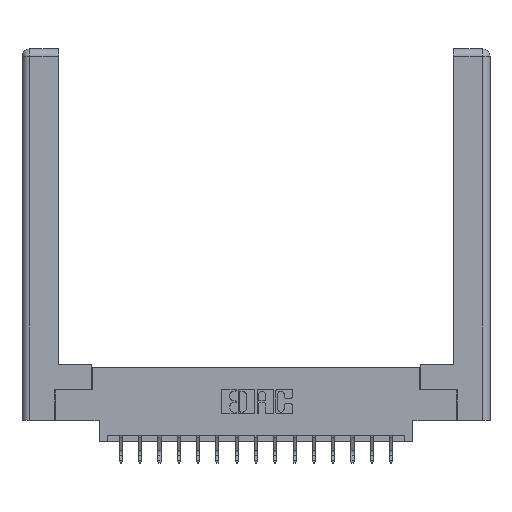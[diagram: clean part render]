
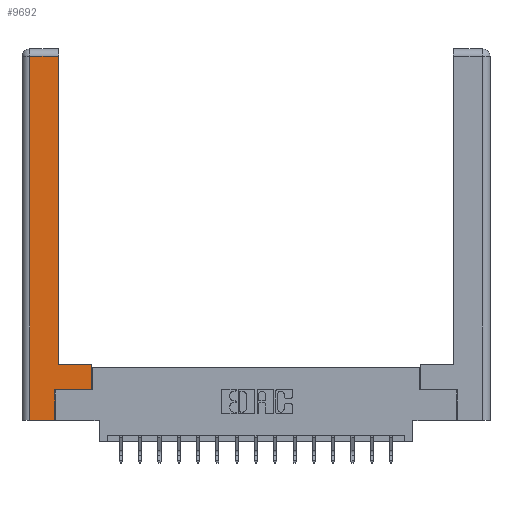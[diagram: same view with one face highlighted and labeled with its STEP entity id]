
A CAD part, top view. The second image highlights one B-rep face of the part: STEP entity #9692.
In plain terms, the highlighted planar face has unit normal (0, 0, 1).
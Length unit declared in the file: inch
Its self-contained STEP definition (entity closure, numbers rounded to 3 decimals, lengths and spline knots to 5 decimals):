
#52 = CARTESIAN_POINT ( 'NONE',  ( 0.265, 0., 0. ) ) ;
#428 = EDGE_CURVE ( 'NONE', #16321, #15442, #13860, .T. ) ;
#539 = DIRECTION ( 'NONE',  ( 0., 0., -1. ) ) ;
#1438 = DIRECTION ( 'NONE',  ( 0., -1., 0. ) ) ;
#1525 = ORIENTED_EDGE ( 'NONE', *, *, #7905, .T. ) ;
#1651 = LINE ( 'NONE', #9757, #3205 ) ;
#1664 = LINE ( 'NONE', #52, #14584 ) ;
#1734 = CARTESIAN_POINT ( 'NONE',  ( 0.565, 0.245, 0. ) ) ;
#1811 = ORIENTED_EDGE ( 'NONE', *, *, #12662, .T. ) ;
#2428 = LINE ( 'NONE', #14267, #14253 ) ;
#2447 = VECTOR ( 'NONE', #12375, 39.37008 ) ;
#2627 = CARTESIAN_POINT ( 'NONE',  ( 0.565, 0.45, 0. ) ) ;
#3205 = VECTOR ( 'NONE', #1438, 39.37008 ) ;
#4074 = EDGE_CURVE ( 'NONE', #4400, #7599, #17051, .T. ) ;
#4400 = VERTEX_POINT ( 'NONE', #11899 ) ;
#4443 = DIRECTION ( 'NONE',  ( -1., 0., 0. ) ) ;
#4630 = CARTESIAN_POINT ( 'NONE',  ( 0.0615, 2.94, 0. ) ) ;
#4712 = EDGE_CURVE ( 'NONE', #17273, #7782, #1664, .T. ) ;
#5134 = CARTESIAN_POINT ( 'NONE',  ( 0.265, 0., 0. ) ) ;
#5208 = CARTESIAN_POINT ( 'NONE',  ( 0.265, 0.245, 0. ) ) ;
#5250 = DIRECTION ( 'NONE',  ( 0., 1., 0. ) ) ;
#5456 = DIRECTION ( 'NONE',  ( -1., 0., 0. ) ) ;
#5463 = ORIENTED_EDGE ( 'NONE', *, *, #17715, .T. ) ;
#5512 = DIRECTION ( 'NONE',  ( 1., 0., 0. ) ) ;
#5730 = CARTESIAN_POINT ( 'NONE',  ( 0.295, 2.94, 0. ) ) ;
#6116 = EDGE_CURVE ( 'NONE', #8384, #17273, #1651, .T. ) ;
#7367 = PLANE ( 'NONE',  #17929 ) ;
#7398 = VECTOR ( 'NONE', #14943, 39.37008 ) ;
#7599 = VERTEX_POINT ( 'NONE', #14137 ) ;
#7782 = VERTEX_POINT ( 'NONE', #5134 ) ;
#7905 = EDGE_CURVE ( 'NONE', #15442, #4400, #14694, .T. ) ;
#8384 = VERTEX_POINT ( 'NONE', #4630 ) ;
#8608 = CARTESIAN_POINT ( 'NONE',  ( 0.0615, 0., 0. ) ) ;
#9020 = VECTOR ( 'NONE', #5250, 39.37008 ) ;
#9692 = ADVANCED_FACE ( 'NONE', ( #17755 ), #7367, .F. ) ;
#9757 = CARTESIAN_POINT ( 'NONE',  ( 0.0615, 0., 0. ) ) ;
#9972 = ORIENTED_EDGE ( 'NONE', *, *, #4074, .T. ) ;
#10035 = ORIENTED_EDGE ( 'NONE', *, *, #6116, .T. ) ;
#10156 = CARTESIAN_POINT ( 'NONE',  ( 0., 0., 0. ) ) ;
#10360 = ORIENTED_EDGE ( 'NONE', *, *, #4712, .T. ) ;
#10824 = ORIENTED_EDGE ( 'NONE', *, *, #17910, .T. ) ;
#10850 = CARTESIAN_POINT ( 'NONE',  ( 0.295, 3., 0. ) ) ;
#10859 = CARTESIAN_POINT ( 'NONE',  ( 0.265, 0.245, 0. ) ) ;
#11100 = LINE ( 'NONE', #10850, #7398 ) ;
#11562 = VECTOR ( 'NONE', #5456, 39.37008 ) ;
#11899 = CARTESIAN_POINT ( 'NONE',  ( 0.565, 0.45, 0. ) ) ;
#12375 = DIRECTION ( 'NONE',  ( 0., 1., 0. ) ) ;
#12538 = CARTESIAN_POINT ( 'NONE',  ( 0.565, 0.245, 0. ) ) ;
#12662 = EDGE_CURVE ( 'NONE', #7599, #14793, #11100, .T. ) ;
#12710 = EDGE_LOOP ( 'NONE', ( #1811, #10824, #10035, #10360, #5463, #17645, #1525, #9972 ) ) ;
#13677 = CARTESIAN_POINT ( 'NONE',  ( 0.295, 0.45, 0. ) ) ;
#13860 = LINE ( 'NONE', #12538, #17180 ) ;
#13935 = DIRECTION ( 'NONE',  ( 1., 0., 0. ) ) ;
#14041 = LINE ( 'NONE', #10859, #2447 ) ;
#14137 = CARTESIAN_POINT ( 'NONE',  ( 0.295, 0.45, 0. ) ) ;
#14253 = VECTOR ( 'NONE', #4443, 39.37008 ) ;
#14267 = CARTESIAN_POINT ( 'NONE',  ( 0.0615, 2.94, 0. ) ) ;
#14584 = VECTOR ( 'NONE', #5512, 39.37008 ) ;
#14694 = LINE ( 'NONE', #2627, #9020 ) ;
#14793 = VERTEX_POINT ( 'NONE', #5730 ) ;
#14943 = DIRECTION ( 'NONE',  ( 0., 1., 0. ) ) ;
#15442 = VERTEX_POINT ( 'NONE', #1734 ) ;
#15773 = DIRECTION ( 'NONE',  ( -1., 0., 0. ) ) ;
#16321 = VERTEX_POINT ( 'NONE', #5208 ) ;
#17051 = LINE ( 'NONE', #13677, #11562 ) ;
#17180 = VECTOR ( 'NONE', #13935, 39.37008 ) ;
#17273 = VERTEX_POINT ( 'NONE', #8608 ) ;
#17645 = ORIENTED_EDGE ( 'NONE', *, *, #428, .T. ) ;
#17715 = EDGE_CURVE ( 'NONE', #7782, #16321, #14041, .T. ) ;
#17755 = FACE_OUTER_BOUND ( 'NONE', #12710, .T. ) ;
#17910 = EDGE_CURVE ( 'NONE', #14793, #8384, #2428, .T. ) ;
#17929 = AXIS2_PLACEMENT_3D ( 'NONE', #10156, #539, #15773 ) ;
